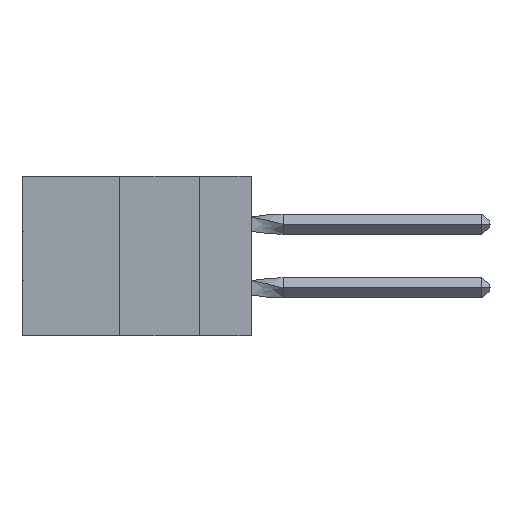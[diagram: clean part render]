
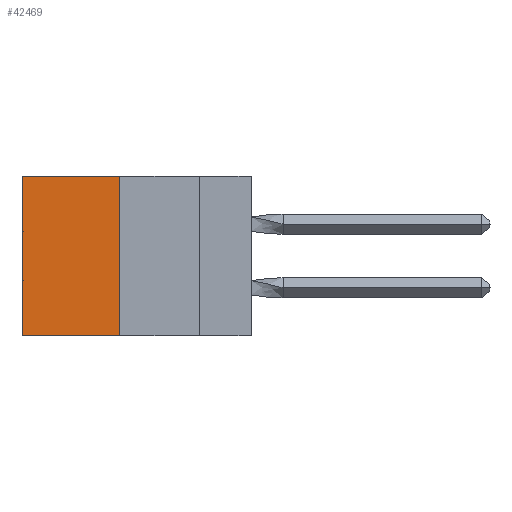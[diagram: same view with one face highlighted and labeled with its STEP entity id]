
A CAD part, left-side view. The second image highlights one B-rep face of the part: STEP entity #42469.
In plain terms, the highlighted planar face has unit normal (-1, 0, 0).
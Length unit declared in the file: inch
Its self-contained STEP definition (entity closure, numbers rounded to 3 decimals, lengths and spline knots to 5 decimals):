
#1860 = DIRECTION ( 'NONE',  ( 0., 1., 0. ) ) ;
#1940 = ORIENTED_EDGE ( 'NONE', *, *, #39115, .T. ) ;
#3059 = LINE ( 'NONE', #31487, #24963 ) ;
#6195 = VERTEX_POINT ( 'NONE', #7893 ) ;
#6295 = LINE ( 'NONE', #25018, #15155 ) ;
#7893 = CARTESIAN_POINT ( 'NONE',  ( 0.305, 0.413, 0. ) ) ;
#9649 = CARTESIAN_POINT ( 'NONE',  ( 0.305, 0.413, -0.5 ) ) ;
#9830 = DIRECTION ( 'NONE',  ( 0., 0., -1. ) ) ;
#10084 = VECTOR ( 'NONE', #19237, 39.37008 ) ;
#10218 = VECTOR ( 'NONE', #1860, 39.37008 ) ;
#11057 = FACE_OUTER_BOUND ( 'NONE', #23897, .T. ) ;
#11827 = CARTESIAN_POINT ( 'NONE',  ( 0.305, 0.413, -0.5 ) ) ;
#12715 = DIRECTION ( 'NONE',  ( 0., 0., -1. ) ) ;
#13943 = ORIENTED_EDGE ( 'NONE', *, *, #35372, .T. ) ;
#14941 = ORIENTED_EDGE ( 'NONE', *, *, #20292, .F. ) ;
#15155 = VECTOR ( 'NONE', #9830, 39.37008 ) ;
#15730 = CARTESIAN_POINT ( 'NONE',  ( 0.305, 0.413, 0. ) ) ;
#19237 = DIRECTION ( 'NONE',  ( 0., 1., 0. ) ) ;
#20292 = EDGE_CURVE ( 'NONE', #34484, #46322, #25033, .T. ) ;
#21346 = LINE ( 'NONE', #15730, #10084 ) ;
#23897 = EDGE_LOOP ( 'NONE', ( #13943, #14941, #45221, #1940 ) ) ;
#24963 = VECTOR ( 'NONE', #12715, 39.37008 ) ;
#25018 = CARTESIAN_POINT ( 'NONE',  ( 0.305, 0.72, -0.5 ) ) ;
#25033 = LINE ( 'NONE', #9649, #10218 ) ;
#30635 = PLANE ( 'NONE',  #42423 ) ;
#31487 = CARTESIAN_POINT ( 'NONE',  ( 0.305, 0.413, -0.5 ) ) ;
#31957 = VERTEX_POINT ( 'NONE', #47481 ) ;
#32938 = CARTESIAN_POINT ( 'NONE',  ( 0.305, 0.72, -0.5 ) ) ;
#34484 = VERTEX_POINT ( 'NONE', #36896 ) ;
#35372 = EDGE_CURVE ( 'NONE', #31957, #46322, #6295, .T. ) ;
#36896 = CARTESIAN_POINT ( 'NONE',  ( 0.305, 0.413, -0.5 ) ) ;
#37827 = DIRECTION ( 'NONE',  ( 0., 0., -1. ) ) ;
#39115 = EDGE_CURVE ( 'NONE', #6195, #31957, #21346, .T. ) ;
#42165 = DIRECTION ( 'NONE',  ( 1., 0., 0. ) ) ;
#42423 = AXIS2_PLACEMENT_3D ( 'NONE', #11827, #42165, #37827 ) ;
#42469 = ADVANCED_FACE ( 'NONE', ( #11057 ), #30635, .F. ) ;
#45221 = ORIENTED_EDGE ( 'NONE', *, *, #48291, .F. ) ;
#46322 = VERTEX_POINT ( 'NONE', #32938 ) ;
#47481 = CARTESIAN_POINT ( 'NONE',  ( 0.305, 0.72, 0. ) ) ;
#48291 = EDGE_CURVE ( 'NONE', #6195, #34484, #3059, .T. ) ;
